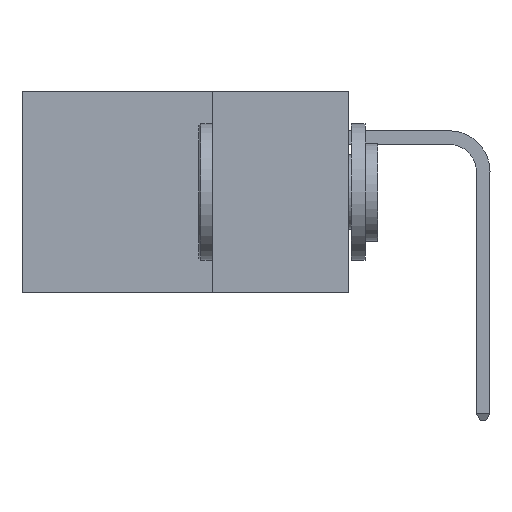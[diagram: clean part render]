
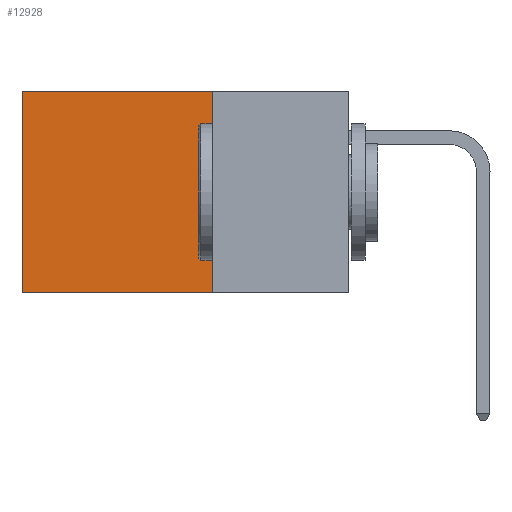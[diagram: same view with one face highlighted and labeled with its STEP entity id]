
A CAD part, left-side view. The second image highlights one B-rep face of the part: STEP entity #12928.
In plain terms, the highlighted planar face has unit normal (-1, 0, 0).
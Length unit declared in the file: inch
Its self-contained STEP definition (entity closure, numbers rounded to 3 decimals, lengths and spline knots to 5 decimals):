
#806 = ORIENTED_EDGE ( 'NONE', *, *, #3810, .F. ) ;
#3334 = VECTOR ( 'NONE', #27473, 39.37008 ) ;
#3810 = EDGE_CURVE ( 'NONE', #6742, #21144, #12062, .T. ) ;
#4239 = CARTESIAN_POINT ( 'NONE',  ( 0.2875, 0.25, -0.37 ) ) ;
#6071 = FACE_OUTER_BOUND ( 'NONE', #26535, .T. ) ;
#6742 = VERTEX_POINT ( 'NONE', #4239 ) ;
#7311 = CARTESIAN_POINT ( 'NONE',  ( 0.2875, 0.25, 0. ) ) ;
#8741 = VERTEX_POINT ( 'NONE', #28506 ) ;
#10410 = LINE ( 'NONE', #32571, #3334 ) ;
#11656 = CARTESIAN_POINT ( 'NONE',  ( 0.2875, 0.6, -0.37 ) ) ;
#12062 = LINE ( 'NONE', #19924, #25260 ) ;
#12553 = PLANE ( 'NONE',  #22974 ) ;
#12928 = ADVANCED_FACE ( 'NONE', ( #6071 ), #12553, .F. ) ;
#13384 = VERTEX_POINT ( 'NONE', #19789 ) ;
#16873 = VECTOR ( 'NONE', #28839, 39.37008 ) ;
#17304 = DIRECTION ( 'NONE',  ( 0., 1., 0. ) ) ;
#17997 = DIRECTION ( 'NONE',  ( 0., 0., -1. ) ) ;
#18280 = CARTESIAN_POINT ( 'NONE',  ( 0.2875, 0.6, 0. ) ) ;
#19742 = DIRECTION ( 'NONE',  ( 0., 0., -1. ) ) ;
#19789 = CARTESIAN_POINT ( 'NONE',  ( 0.2875, 0.6, 0. ) ) ;
#19855 = EDGE_CURVE ( 'NONE', #8741, #6742, #31886, .T. ) ;
#19924 = CARTESIAN_POINT ( 'NONE',  ( 0.2875, 0.25, -0.37 ) ) ;
#21144 = VERTEX_POINT ( 'NONE', #11656 ) ;
#22254 = ORIENTED_EDGE ( 'NONE', *, *, #19855, .F. ) ;
#22487 = EDGE_CURVE ( 'NONE', #8741, #13384, #10410, .T. ) ;
#22974 = AXIS2_PLACEMENT_3D ( 'NONE', #7311, #33607, #17997 ) ;
#23868 = LINE ( 'NONE', #18280, #16873 ) ;
#24892 = ORIENTED_EDGE ( 'NONE', *, *, #25744, .T. ) ;
#24977 = VECTOR ( 'NONE', #19742, 39.37008 ) ;
#25260 = VECTOR ( 'NONE', #17304, 39.37008 ) ;
#25744 = EDGE_CURVE ( 'NONE', #13384, #21144, #23868, .T. ) ;
#25857 = ORIENTED_EDGE ( 'NONE', *, *, #22487, .T. ) ;
#26535 = EDGE_LOOP ( 'NONE', ( #24892, #806, #22254, #25857 ) ) ;
#27473 = DIRECTION ( 'NONE',  ( 0., 1., 0. ) ) ;
#27546 = CARTESIAN_POINT ( 'NONE',  ( 0.2875, 0.25, 0. ) ) ;
#28506 = CARTESIAN_POINT ( 'NONE',  ( 0.2875, 0.25, 0. ) ) ;
#28839 = DIRECTION ( 'NONE',  ( 0., 0., -1. ) ) ;
#31886 = LINE ( 'NONE', #27546, #24977 ) ;
#32571 = CARTESIAN_POINT ( 'NONE',  ( 0.2875, 0.25, 0. ) ) ;
#33607 = DIRECTION ( 'NONE',  ( 1., 0., 0. ) ) ;
